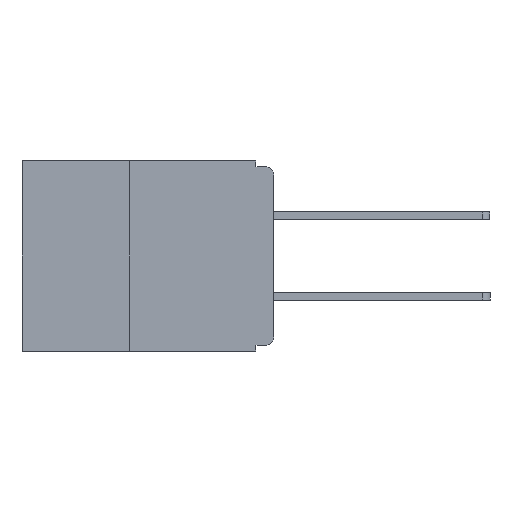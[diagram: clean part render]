
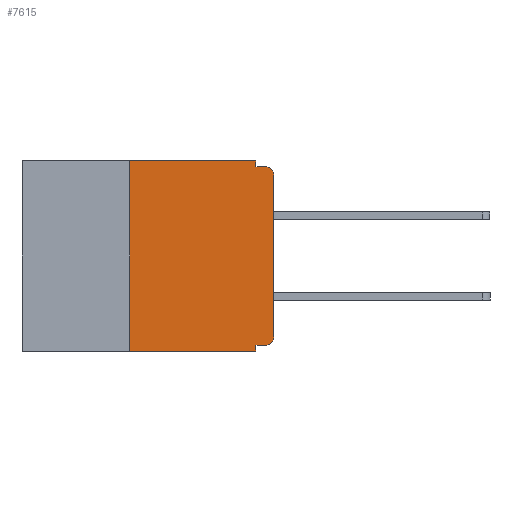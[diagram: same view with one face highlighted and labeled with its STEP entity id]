
A CAD part, left-side view. The second image highlights one B-rep face of the part: STEP entity #7615.
In plain terms, the highlighted planar face has unit normal (-1, 0, 0).
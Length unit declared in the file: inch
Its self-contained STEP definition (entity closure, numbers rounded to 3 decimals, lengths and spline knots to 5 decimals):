
#679 = LINE ( 'NONE', #7338, #28387 ) ;
#836 = CARTESIAN_POINT ( 'NONE',  ( 0., 0., 0. ) ) ;
#1029 = ORIENTED_EDGE ( 'NONE', *, *, #22936, .F. ) ;
#1335 = CARTESIAN_POINT ( 'NONE',  ( 0., 0.437, -0.33 ) ) ;
#1449 = DIRECTION ( 'NONE',  ( 0., 0., -1. ) ) ;
#2748 = DIRECTION ( 'NONE',  ( -1., 0., 0. ) ) ;
#3046 = PLANE ( 'NONE',  #3904 ) ;
#3154 = EDGE_CURVE ( 'NONE', #14675, #31995, #4479, .T. ) ;
#3776 = DIRECTION ( 'NONE',  ( -1., 0., 0. ) ) ;
#3904 = AXIS2_PLACEMENT_3D ( 'NONE', #21788, #5754, #24506 ) ;
#4019 = ORIENTED_EDGE ( 'NONE', *, *, #19857, .T. ) ;
#4032 = FACE_OUTER_BOUND ( 'NONE', #14369, .T. ) ;
#4192 = VECTOR ( 'NONE', #22286, 39.37008 ) ;
#4459 = ORIENTED_EDGE ( 'NONE', *, *, #23065, .T. ) ;
#4479 = LINE ( 'NONE', #6911, #10828 ) ;
#4760 = VERTEX_POINT ( 'NONE', #34542 ) ;
#4798 = CARTESIAN_POINT ( 'NONE',  ( 0., 0.015, -0.01 ) ) ;
#5130 = CIRCLE ( 'NONE', #14599, 0.015 ) ;
#5202 = DIRECTION ( 'NONE',  ( 0., -1., 0. ) ) ;
#5754 = DIRECTION ( 'NONE',  ( 1., 0., 0. ) ) ;
#6143 = ORIENTED_EDGE ( 'NONE', *, *, #11032, .T. ) ;
#6911 = CARTESIAN_POINT ( 'NONE',  ( 0., 0.437, 0. ) ) ;
#7338 = CARTESIAN_POINT ( 'NONE',  ( 0., 0.25, -0.33 ) ) ;
#7615 = ADVANCED_FACE ( 'NONE', ( #4032 ), #3046, .F. ) ;
#7934 = VERTEX_POINT ( 'NONE', #9768 ) ;
#8230 = VERTEX_POINT ( 'NONE', #8284 ) ;
#8284 = CARTESIAN_POINT ( 'NONE',  ( 0., 0.015, -0.32 ) ) ;
#8607 = VECTOR ( 'NONE', #20090, 39.37008 ) ;
#9240 = LINE ( 'NONE', #14275, #21764 ) ;
#9768 = CARTESIAN_POINT ( 'NONE',  ( 0., 0.25, -0.33 ) ) ;
#10660 = CARTESIAN_POINT ( 'NONE',  ( 0., 0.031, 0. ) ) ;
#10704 = VERTEX_POINT ( 'NONE', #17111 ) ;
#10828 = VECTOR ( 'NONE', #5202, 39.37008 ) ;
#11032 = EDGE_CURVE ( 'NONE', #4760, #28549, #5130, .T. ) ;
#11057 = DIRECTION ( 'NONE',  ( 0., 1., 0. ) ) ;
#11475 = VECTOR ( 'NONE', #1449, 39.37008 ) ;
#12282 = CARTESIAN_POINT ( 'NONE',  ( 0., 0.25, 0. ) ) ;
#13062 = LINE ( 'NONE', #836, #4192 ) ;
#13888 = CIRCLE ( 'NONE', #27989, 0.015 ) ;
#14275 = CARTESIAN_POINT ( 'NONE',  ( 0., 0., -0.01 ) ) ;
#14369 = EDGE_LOOP ( 'NONE', ( #4459, #6143, #34573, #1029, #17003, #22004, #4019, #34154, #15423, #18688 ) ) ;
#14599 = AXIS2_PLACEMENT_3D ( 'NONE', #18813, #2748, #21490 ) ;
#14634 = VERTEX_POINT ( 'NONE', #22748 ) ;
#14675 = VERTEX_POINT ( 'NONE', #12282 ) ;
#15423 = ORIENTED_EDGE ( 'NONE', *, *, #16282, .F. ) ;
#15584 = VECTOR ( 'NONE', #32023, 39.37008 ) ;
#16282 = EDGE_CURVE ( 'NONE', #8230, #18593, #26608, .T. ) ;
#17003 = ORIENTED_EDGE ( 'NONE', *, *, #3154, .F. ) ;
#17111 = CARTESIAN_POINT ( 'NONE',  ( 0., 0.031, -0.01 ) ) ;
#17545 = CARTESIAN_POINT ( 'NONE',  ( 0., 0.031, -0.33 ) ) ;
#18565 = CARTESIAN_POINT ( 'NONE',  ( 0., 0.031, -0.32 ) ) ;
#18593 = VERTEX_POINT ( 'NONE', #18565 ) ;
#18688 = ORIENTED_EDGE ( 'NONE', *, *, #30150, .T. ) ;
#18813 = CARTESIAN_POINT ( 'NONE',  ( 0., 0.015, -0.025 ) ) ;
#18961 = CARTESIAN_POINT ( 'NONE',  ( 0., 0.031, 0. ) ) ;
#19470 = VECTOR ( 'NONE', #11057, 39.37008 ) ;
#19810 = CARTESIAN_POINT ( 'NONE',  ( 0., 0.015, -0.305 ) ) ;
#19857 = EDGE_CURVE ( 'NONE', #7934, #14634, #22009, .T. ) ;
#20090 = DIRECTION ( 'NONE',  ( 0., -1., 0. ) ) ;
#21490 = DIRECTION ( 'NONE',  ( 0., 0., -1. ) ) ;
#21702 = EDGE_CURVE ( 'NONE', #18593, #14634, #32795, .T. ) ;
#21764 = VECTOR ( 'NONE', #24969, 39.37008 ) ;
#21788 = CARTESIAN_POINT ( 'NONE',  ( 0., 0.437, 0. ) ) ;
#22004 = ORIENTED_EDGE ( 'NONE', *, *, #32414, .F. ) ;
#22009 = LINE ( 'NONE', #1335, #8607 ) ;
#22286 = DIRECTION ( 'NONE',  ( 0., 0., 1. ) ) ;
#22505 = DIRECTION ( 'NONE',  ( 0., 0., -1. ) ) ;
#22748 = CARTESIAN_POINT ( 'NONE',  ( 0., 0.031, -0.33 ) ) ;
#22936 = EDGE_CURVE ( 'NONE', #31995, #10704, #28933, .T. ) ;
#23065 = EDGE_CURVE ( 'NONE', #26394, #4760, #13062, .T. ) ;
#24506 = DIRECTION ( 'NONE',  ( 0., 0., -1. ) ) ;
#24969 = DIRECTION ( 'NONE',  ( 0., -1., 0. ) ) ;
#26394 = VERTEX_POINT ( 'NONE', #33116 ) ;
#26608 = LINE ( 'NONE', #29713, #19470 ) ;
#27989 = AXIS2_PLACEMENT_3D ( 'NONE', #19810, #3776, #22505 ) ;
#28387 = VECTOR ( 'NONE', #28785, 39.37008 ) ;
#28549 = VERTEX_POINT ( 'NONE', #4798 ) ;
#28785 = DIRECTION ( 'NONE',  ( 0., 0., 1. ) ) ;
#28933 = LINE ( 'NONE', #10660, #15584 ) ;
#29713 = CARTESIAN_POINT ( 'NONE',  ( 0., 0., -0.32 ) ) ;
#30095 = EDGE_CURVE ( 'NONE', #10704, #28549, #9240, .T. ) ;
#30150 = EDGE_CURVE ( 'NONE', #8230, #26394, #13888, .T. ) ;
#31995 = VERTEX_POINT ( 'NONE', #18961 ) ;
#32023 = DIRECTION ( 'NONE',  ( 0., 0., -1. ) ) ;
#32414 = EDGE_CURVE ( 'NONE', #7934, #14675, #679, .T. ) ;
#32795 = LINE ( 'NONE', #17545, #11475 ) ;
#33116 = CARTESIAN_POINT ( 'NONE',  ( 0., 0., -0.305 ) ) ;
#34154 = ORIENTED_EDGE ( 'NONE', *, *, #21702, .F. ) ;
#34542 = CARTESIAN_POINT ( 'NONE',  ( 0., 0., -0.025 ) ) ;
#34573 = ORIENTED_EDGE ( 'NONE', *, *, #30095, .F. ) ;
